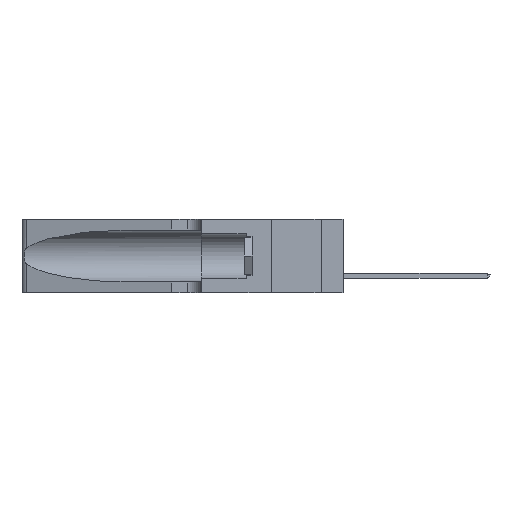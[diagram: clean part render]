
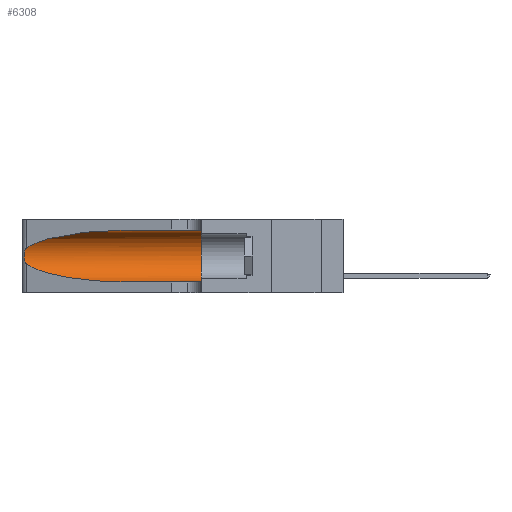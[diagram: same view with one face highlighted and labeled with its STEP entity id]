
A CAD part, left-side view. The second image highlights one B-rep face of the part: STEP entity #6308.
In plain terms, the highlighted cylindrical face has radius 3.308 mm (diameter 6.617 mm), a partial arc.
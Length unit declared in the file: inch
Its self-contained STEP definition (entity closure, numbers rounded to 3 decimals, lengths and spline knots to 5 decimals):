
#141 = CARTESIAN_POINT ( 'NONE',  ( 0.1305, 0.72297, 0.31525 ) ) ;
#1323 = ORIENTED_EDGE ( 'NONE', *, *, #15714, .F. ) ;
#1522 = CARTESIAN_POINT ( 'NONE',  ( 0.1305, 0.72297, 0.05475 ) ) ;
#2137 = CARTESIAN_POINT ( 'NONE',  ( 0.25854, 1.2359, 0.20912 ) ) ;
#2388 = CARTESIAN_POINT ( 'NONE',  ( 0.26017, 1.23833, 0.17102 ) ) ;
#2747 = CARTESIAN_POINT ( 'NONE',  ( 0.1305, 1.61858, 0.05475 ) ) ;
#2848 = CARTESIAN_POINT ( 'NONE',  ( 0.25789, 1.23486, 0.15765 ) ) ;
#4435 = LINE ( 'NONE', #7651, #30411 ) ;
#5118 = CARTESIAN_POINT ( 'NONE',  ( 0.1305, 0.35, 0.185 ) ) ;
#5714 = CARTESIAN_POINT ( 'NONE',  ( 0.25487, 1.22718, 0.14631 ) ) ;
#6308 = ADVANCED_FACE ( 'NONE', ( #31926 ), #35777, .F. ) ;
#6547 = EDGE_CURVE ( 'NONE', #13997, #32893, #30709, .T. ) ;
#6571 = EDGE_CURVE ( 'NONE', #32893, #27366, #31326, .T. ) ;
#7651 = CARTESIAN_POINT ( 'NONE',  ( 0.1305, 1.61858, 0.31525 ) ) ;
#7929 = CARTESIAN_POINT ( 'NONE',  ( 0.26075, 1.23896, 0.19203 ) ) ;
#8491 = ORIENTED_EDGE ( 'NONE', *, *, #23132, .T. ) ;
#9133 = DIRECTION ( 'NONE',  ( 0., -1., 0. ) ) ;
#9899 = CARTESIAN_POINT ( 'NONE',  ( 0.1305, 0.72297, 0.31525 ) ) ;
#10168 = CARTESIAN_POINT ( 'NONE',  ( 0.1305, 1.61858, 0.185 ) ) ;
#10868 = AXIS2_PLACEMENT_3D ( 'NONE', #10168, #32407, #35577 ) ;
#11932 = CARTESIAN_POINT ( 'NONE',  ( 0.25487, 1.22718, 0.14631 ) ) ;
#12678 = VERTEX_POINT ( 'NONE', #16801 ) ;
#13997 = VERTEX_POINT ( 'NONE', #14302 ) ;
#14302 = CARTESIAN_POINT ( 'NONE',  ( 0.25487, 1.22718, 0.22369 ) ) ;
#14331 = ORIENTED_EDGE ( 'NONE', *, *, #33540, .T. ) ;
#15625 = ORIENTED_EDGE ( 'NONE', *, *, #6547, .T. ) ;
#15714 = EDGE_CURVE ( 'NONE', #22153, #12678, #4435, .T. ) ;
#16134 = CARTESIAN_POINT ( 'NONE',  ( 0.25639, 1.23184, 0.21858 ) ) ;
#16371 = CARTESIAN_POINT ( 'NONE',  ( 0.25787, 1.23484, 0.2124 ) ) ;
#16604 = CARTESIAN_POINT ( 'NONE',  ( 0.25555, 1.22993, 0.14849 ) ) ;
#16801 = CARTESIAN_POINT ( 'NONE',  ( 0.1305, 0.35, 0.31525 ) ) ;
#21506 = ORIENTED_EDGE ( 'NONE', *, *, #6571, .T. ) ;
#21586 = AXIS2_PLACEMENT_3D ( 'NONE', #5118, #24785, #27161 ) ;
#21670 = EDGE_LOOP ( 'NONE', ( #14331, #15625, #21506, #8491, #34316, #1323 ) ) ;
#21820 = CARTESIAN_POINT ( 'NONE',  ( 0.26018, 1.23835, 0.19895 ) ) ;
#22153 = VERTEX_POINT ( 'NONE', #9899 ) ;
#22181 = CARTESIAN_POINT ( 'NONE',  ( 0.18966, 0.96281, 0.31525 ) ) ;
#22620 = CARTESIAN_POINT ( 'NONE',  ( 0.25856, 1.23593, 0.16098 ) ) ;
#23132 = EDGE_CURVE ( 'NONE', #27366, #27334, #28156, .T. ) ;
#23202 = CARTESIAN_POINT ( 'NONE',  ( 0.2373, 1.15595, 0.08982 ) ) ;
#24785 = DIRECTION ( 'NONE',  ( 0., 1., 0. ) ) ;
#24899 = CARTESIAN_POINT ( 'NONE',  ( 0.25487, 1.22718, 0.14631 ) ) ;
#27161 = DIRECTION ( 'NONE',  ( 0., 0., 1. ) ) ;
#27334 = VERTEX_POINT ( 'NONE', #31769 ) ;
#27366 = VERTEX_POINT ( 'NONE', #1522 ) ;
#27881 = CARTESIAN_POINT ( 'NONE',  ( 0.2373, 1.15595, 0.28018 ) ) ;
#28156 = LINE ( 'NONE', #2747, #33442 ) ;
#29136 = CARTESIAN_POINT ( 'NONE',  ( 0.1305, 0.72297, 0.05475 ) ) ;
#30411 = VECTOR ( 'NONE', #9133, 39.37008 ) ;
#30709 = B_SPLINE_CURVE_WITH_KNOTS ( 'NONE', 3,
 ( #32884, #33009, #16134, #16371, #2137, #21820, #7929, #36049, #2388, #22620, #2848, #33501, #16604, #24899 ),
 .UNSPECIFIED., .F., .F.,
 ( 4, 2, 2, 2, 2, 2, 4 ),
 ( 0., 0.00027, 0.00053, 0.00107, 0.0016, 0.00187, 0.00214 ),
 .UNSPECIFIED. ) ;
#31010 = CARTESIAN_POINT ( 'NONE',  ( 0.25487, 1.22718, 0.22369 ) ) ;
#31326 =( BOUNDED_CURVE ( )  B_SPLINE_CURVE ( 3, ( #11932, #23202, #31588, #29136 ),
 .UNSPECIFIED., .F., .F. ) 
 B_SPLINE_CURVE_WITH_KNOTS ( ( 4, 4 ),
 ( 3.44316, 4.71239 ),
 .UNSPECIFIED. ) 
 CURVE ( )  GEOMETRIC_REPRESENTATION_ITEM ( )  RATIONAL_B_SPLINE_CURVE ( ( 1., 0.87, 0.87, 1. ) ) 
 REPRESENTATION_ITEM ( '' )  );
#31588 = CARTESIAN_POINT ( 'NONE',  ( 0.18966, 0.96281, 0.05475 ) ) ;
#31769 = CARTESIAN_POINT ( 'NONE',  ( 0.1305, 0.35, 0.05475 ) ) ;
#31926 = FACE_OUTER_BOUND ( 'NONE', #21670, .T. ) ;
#32381 = CIRCLE ( 'NONE', #21586, 0.13025 ) ;
#32407 = DIRECTION ( 'NONE',  ( 0., -1., 0. ) ) ;
#32884 = CARTESIAN_POINT ( 'NONE',  ( 0.25487, 1.22718, 0.22369 ) ) ;
#32893 = VERTEX_POINT ( 'NONE', #5714 ) ;
#32953 =( BOUNDED_CURVE ( )  B_SPLINE_CURVE ( 3, ( #141, #22181, #27881, #31010 ),
 .UNSPECIFIED., .F., .F. ) 
 B_SPLINE_CURVE_WITH_KNOTS ( ( 4, 4 ),
 ( 1.5708, 2.84003 ),
 .UNSPECIFIED. ) 
 CURVE ( )  GEOMETRIC_REPRESENTATION_ITEM ( )  RATIONAL_B_SPLINE_CURVE ( ( 1., 0.87, 0.87, 1. ) ) 
 REPRESENTATION_ITEM ( '' )  );
#33009 = CARTESIAN_POINT ( 'NONE',  ( 0.25555, 1.22994, 0.2215 ) ) ;
#33442 = VECTOR ( 'NONE', #35564, 39.37008 ) ;
#33472 = EDGE_CURVE ( 'NONE', #12678, #27334, #32381, .T. ) ;
#33501 = CARTESIAN_POINT ( 'NONE',  ( 0.25639, 1.23186, 0.15144 ) ) ;
#33540 = EDGE_CURVE ( 'NONE', #22153, #13997, #32953, .T. ) ;
#34316 = ORIENTED_EDGE ( 'NONE', *, *, #33472, .F. ) ;
#35564 = DIRECTION ( 'NONE',  ( 0., -1., 0. ) ) ;
#35577 = DIRECTION ( 'NONE',  ( 0., 0., -1. ) ) ;
#35777 = CYLINDRICAL_SURFACE ( 'NONE', #10868, 0.13025 ) ;
#36049 = CARTESIAN_POINT ( 'NONE',  ( 0.26075, 1.23896, 0.178 ) ) ;
